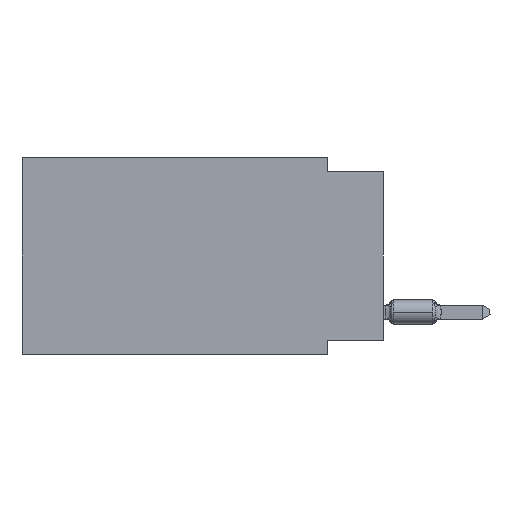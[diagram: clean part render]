
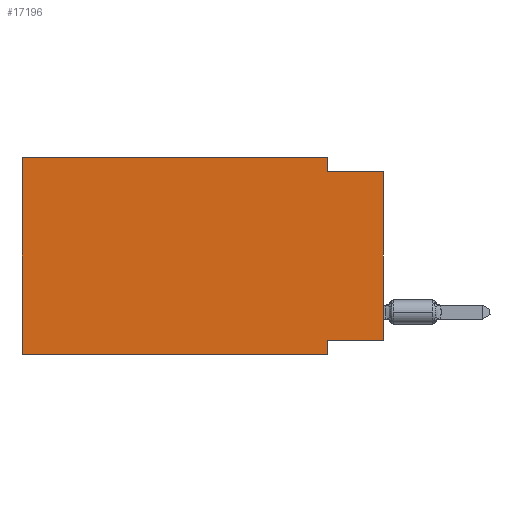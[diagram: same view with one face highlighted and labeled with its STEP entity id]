
A CAD part, left-side view. The second image highlights one B-rep face of the part: STEP entity #17196.
In plain terms, the highlighted planar face has unit normal (-1, 0, 0).
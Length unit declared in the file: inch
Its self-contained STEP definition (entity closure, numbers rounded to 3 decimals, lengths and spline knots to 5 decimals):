
#97 = VERTEX_POINT ( 'NONE', #8118 ) ;
#1012 = ORIENTED_EDGE ( 'NONE', *, *, #23978, .T. ) ;
#1663 = EDGE_CURVE ( 'NONE', #11004, #47392, #39035, .T. ) ;
#2962 = DIRECTION ( 'NONE',  ( 0., -1., 0. ) ) ;
#3385 = EDGE_CURVE ( 'NONE', #59010, #66809, #70715, .T. ) ;
#3425 = VERTEX_POINT ( 'NONE', #47838 ) ;
#4195 = DIRECTION ( 'NONE',  ( 1., 0., 0. ) ) ;
#4338 = CARTESIAN_POINT ( 'NONE',  ( 0., 0., 0. ) ) ;
#5177 = CARTESIAN_POINT ( 'NONE',  ( 0., 0.645, 0. ) ) ;
#8118 = CARTESIAN_POINT ( 'NONE',  ( 0., 0.1, -0.35 ) ) ;
#9992 = VECTOR ( 'NONE', #29795, 39.37008 ) ;
#10431 = LINE ( 'NONE', #4338, #22057 ) ;
#11004 = VERTEX_POINT ( 'NONE', #66930 ) ;
#13477 = ORIENTED_EDGE ( 'NONE', *, *, #22311, .F. ) ;
#14581 = DIRECTION ( 'NONE',  ( 0., 0., -1. ) ) ;
#15162 = EDGE_CURVE ( 'NONE', #25169, #34987, #30895, .T. ) ;
#15664 = DIRECTION ( 'NONE',  ( 0., 0., 1. ) ) ;
#16239 = CARTESIAN_POINT ( 'NONE',  ( 0., 0.1, 0. ) ) ;
#17196 = ADVANCED_FACE ( 'NONE', ( #20304 ), #42812, .F. ) ;
#17459 = EDGE_CURVE ( 'NONE', #34987, #3425, #45895, .T. ) ;
#18872 = VECTOR ( 'NONE', #30217, 39.37008 ) ;
#20304 = FACE_OUTER_BOUND ( 'NONE', #52001, .T. ) ;
#20665 = CARTESIAN_POINT ( 'NONE',  ( 0., 0.645, 0. ) ) ;
#22057 = VECTOR ( 'NONE', #64737, 39.37008 ) ;
#22311 = EDGE_CURVE ( 'NONE', #47392, #97, #30289, .T. ) ;
#23890 = VECTOR ( 'NONE', #35904, 39.37008 ) ;
#23978 = EDGE_CURVE ( 'NONE', #59010, #97, #62746, .T. ) ;
#25169 = VERTEX_POINT ( 'NONE', #16239 ) ;
#26375 = CARTESIAN_POINT ( 'NONE',  ( 0., 0.645, 0. ) ) ;
#26905 = DIRECTION ( 'NONE',  ( 0., 1., 0. ) ) ;
#27276 = ORIENTED_EDGE ( 'NONE', *, *, #52506, .T. ) ;
#29584 = DIRECTION ( 'NONE',  ( 0., 0., -1. ) ) ;
#29795 = DIRECTION ( 'NONE',  ( 0., -1., 0. ) ) ;
#30217 = DIRECTION ( 'NONE',  ( 0., -1., 0. ) ) ;
#30289 = LINE ( 'NONE', #52108, #35824 ) ;
#30749 = AXIS2_PLACEMENT_3D ( 'NONE', #20665, #4195, #14581 ) ;
#30895 = LINE ( 'NONE', #47362, #23890 ) ;
#33053 = VECTOR ( 'NONE', #2962, 39.37008 ) ;
#34987 = VERTEX_POINT ( 'NONE', #58875 ) ;
#35131 = CARTESIAN_POINT ( 'NONE',  ( 0., 0., -0.025 ) ) ;
#35562 = CARTESIAN_POINT ( 'NONE',  ( 0., 0.645, -0.35 ) ) ;
#35824 = VECTOR ( 'NONE', #29584, 39.37008 ) ;
#35904 = DIRECTION ( 'NONE',  ( 0., 0., -1. ) ) ;
#38598 = ORIENTED_EDGE ( 'NONE', *, *, #3385, .F. ) ;
#39035 = LINE ( 'NONE', #48716, #46466 ) ;
#39155 = ORIENTED_EDGE ( 'NONE', *, *, #59070, .F. ) ;
#40022 = VECTOR ( 'NONE', #15664, 39.37008 ) ;
#42812 = PLANE ( 'NONE',  #30749 ) ;
#44499 = CARTESIAN_POINT ( 'NONE',  ( 0., 0.645, -0.35 ) ) ;
#44517 = ORIENTED_EDGE ( 'NONE', *, *, #15162, .F. ) ;
#44802 = ORIENTED_EDGE ( 'NONE', *, *, #17459, .F. ) ;
#45354 = ORIENTED_EDGE ( 'NONE', *, *, #1663, .F. ) ;
#45895 = LINE ( 'NONE', #35131, #33053 ) ;
#46466 = VECTOR ( 'NONE', #26905, 39.37008 ) ;
#47362 = CARTESIAN_POINT ( 'NONE',  ( 0., 0.1, 0. ) ) ;
#47392 = VERTEX_POINT ( 'NONE', #50611 ) ;
#47838 = CARTESIAN_POINT ( 'NONE',  ( 0., 0., -0.025 ) ) ;
#48716 = CARTESIAN_POINT ( 'NONE',  ( 0., 0., -0.325 ) ) ;
#50611 = CARTESIAN_POINT ( 'NONE',  ( 0., 0.1, -0.325 ) ) ;
#52001 = EDGE_LOOP ( 'NONE', ( #27276, #44802, #44517, #39155, #38598, #1012, #13477, #45354 ) ) ;
#52108 = CARTESIAN_POINT ( 'NONE',  ( 0., 0.1, -0.35 ) ) ;
#52506 = EDGE_CURVE ( 'NONE', #11004, #3425, #10431, .T. ) ;
#58381 = LINE ( 'NONE', #63726, #9992 ) ;
#58875 = CARTESIAN_POINT ( 'NONE',  ( 0., 0.1, -0.025 ) ) ;
#59010 = VERTEX_POINT ( 'NONE', #44499 ) ;
#59070 = EDGE_CURVE ( 'NONE', #66809, #25169, #58381, .T. ) ;
#62746 = LINE ( 'NONE', #35562, #18872 ) ;
#63726 = CARTESIAN_POINT ( 'NONE',  ( 0., 0.645, 0. ) ) ;
#64737 = DIRECTION ( 'NONE',  ( 0., 0., 1. ) ) ;
#66809 = VERTEX_POINT ( 'NONE', #5177 ) ;
#66930 = CARTESIAN_POINT ( 'NONE',  ( 0., 0., -0.325 ) ) ;
#70715 = LINE ( 'NONE', #26375, #40022 ) ;
